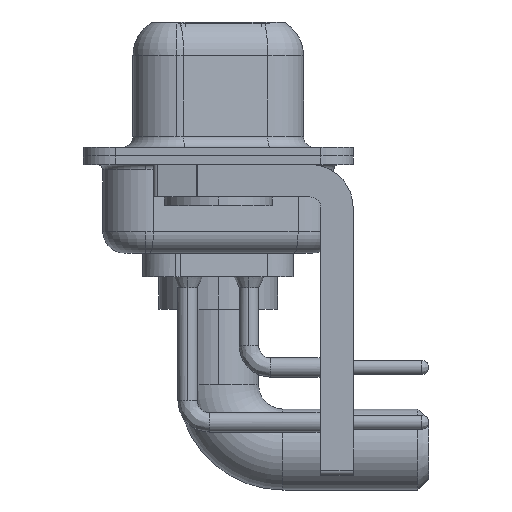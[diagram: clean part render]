
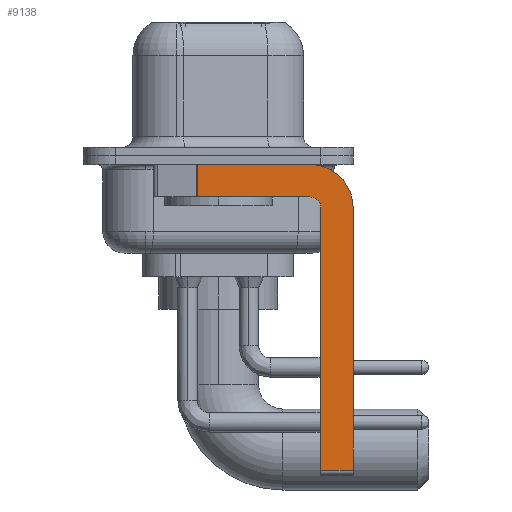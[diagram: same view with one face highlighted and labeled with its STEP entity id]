
A CAD part, left-side view. The second image highlights one B-rep face of the part: STEP entity #9138.
In plain terms, the highlighted planar face has unit normal (-1, 0, 0).
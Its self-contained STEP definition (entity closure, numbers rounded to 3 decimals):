
#435 = CARTESIAN_POINT ( 'NONE',  ( -2.9, -6.25, -2.4 ) ) ;
#586 = AXIS2_PLACEMENT_3D ( 'NONE', #21592, #14474, #12707 ) ;
#688 = VECTOR ( 'NONE', #22884, 1000. ) ;
#944 = CARTESIAN_POINT ( 'NONE',  ( -2.9, 0.978, -1.9 ) ) ;
#1614 = VERTEX_POINT ( 'NONE', #435 ) ;
#1629 = EDGE_CURVE ( 'NONE', #1614, #20230, #9547, .T. ) ;
#2034 = CARTESIAN_POINT ( 'NONE',  ( -2.9, -4.25, -2.4 ) ) ;
#2364 = LINE ( 'NONE', #22265, #22281 ) ;
#2921 = CARTESIAN_POINT ( 'NONE',  ( -2.9, 0.978, -1.9 ) ) ;
#3086 = EDGE_CURVE ( 'NONE', #14313, #6883, #2364, .T. ) ;
#3100 = LINE ( 'NONE', #15648, #688 ) ;
#3863 = CARTESIAN_POINT ( 'NONE',  ( -2.9, -6.25, -2.4 ) ) ;
#4232 = ORIENTED_EDGE ( 'NONE', *, *, #3086, .F. ) ;
#4693 = DIRECTION ( 'NONE',  ( 0., -1., 0. ) ) ;
#4716 = ORIENTED_EDGE ( 'NONE', *, *, #12273, .F. ) ;
#4939 = CARTESIAN_POINT ( 'NONE',  ( -2.9, -4.25, -14.55 ) ) ;
#5197 = CIRCLE ( 'NONE', #21853, 2. ) ;
#5998 = DIRECTION ( 'NONE',  ( 0., 0., -1. ) ) ;
#6318 = EDGE_CURVE ( 'NONE', #11591, #14414, #12734, .T. ) ;
#6357 = CARTESIAN_POINT ( 'NONE',  ( -2.9, 0.978, -0.4 ) ) ;
#6883 = VERTEX_POINT ( 'NONE', #15185 ) ;
#7040 = CARTESIAN_POINT ( 'NONE',  ( -2.9, -4.25, -1.9 ) ) ;
#7110 = AXIS2_PLACEMENT_3D ( 'NONE', #2034, #9254, #7489 ) ;
#7371 = VECTOR ( 'NONE', #9440, 1000. ) ;
#7489 = DIRECTION ( 'NONE',  ( 0., 0., 1. ) ) ;
#7573 = CARTESIAN_POINT ( 'NONE',  ( -2.9, -4.75, -14.55 ) ) ;
#7605 = EDGE_CURVE ( 'NONE', #14313, #14414, #9942, .T. ) ;
#8530 = EDGE_CURVE ( 'NONE', #14307, #11591, #12402, .T. ) ;
#9138 = ADVANCED_FACE ( 'NONE', ( #16151 ), #14369, .F. ) ;
#9254 = DIRECTION ( 'NONE',  ( -1., 0., 0. ) ) ;
#9440 = DIRECTION ( 'NONE',  ( 0., 1., 0. ) ) ;
#9455 = ORIENTED_EDGE ( 'NONE', *, *, #10860, .F. ) ;
#9519 = VERTEX_POINT ( 'NONE', #7573 ) ;
#9547 = LINE ( 'NONE', #3863, #20745 ) ;
#9942 = LINE ( 'NONE', #944, #23328 ) ;
#10139 = EDGE_LOOP ( 'NONE', ( #4232, #22331, #16181, #12250, #9455, #12222, #22493, #4716 ) ) ;
#10860 = EDGE_CURVE ( 'NONE', #9519, #14307, #3100, .T. ) ;
#11591 = VERTEX_POINT ( 'NONE', #7040 ) ;
#11693 = CARTESIAN_POINT ( 'NONE',  ( -2.9, -4.75, -2.4 ) ) ;
#12222 = ORIENTED_EDGE ( 'NONE', *, *, #22833, .T. ) ;
#12250 = ORIENTED_EDGE ( 'NONE', *, *, #8530, .F. ) ;
#12273 = EDGE_CURVE ( 'NONE', #6883, #1614, #5197, .T. ) ;
#12402 = CIRCLE ( 'NONE', #7110, 0.5 ) ;
#12707 = DIRECTION ( 'NONE',  ( 0., 0., -1. ) ) ;
#12734 = LINE ( 'NONE', #21982, #7371 ) ;
#13259 = DIRECTION ( 'NONE',  ( 0., -1., 0. ) ) ;
#13646 = DIRECTION ( 'NONE',  ( 1., 0., 0. ) ) ;
#14307 = VERTEX_POINT ( 'NONE', #11693 ) ;
#14313 = VERTEX_POINT ( 'NONE', #6357 ) ;
#14369 = PLANE ( 'NONE',  #586 ) ;
#14414 = VERTEX_POINT ( 'NONE', #2921 ) ;
#14474 = DIRECTION ( 'NONE',  ( 1., 0., 0. ) ) ;
#14510 = CARTESIAN_POINT ( 'NONE',  ( -2.9, -6.25, -14.55 ) ) ;
#15185 = CARTESIAN_POINT ( 'NONE',  ( -2.9, -4.25, -0.4 ) ) ;
#15614 = DIRECTION ( 'NONE',  ( 0., 0., -1. ) ) ;
#15648 = CARTESIAN_POINT ( 'NONE',  ( -2.9, -4.75, -14.8 ) ) ;
#16151 = FACE_OUTER_BOUND ( 'NONE', #10139, .T. ) ;
#16181 = ORIENTED_EDGE ( 'NONE', *, *, #6318, .F. ) ;
#17606 = LINE ( 'NONE', #4939, #18747 ) ;
#18747 = VECTOR ( 'NONE', #4693, 1000. ) ;
#20230 = VERTEX_POINT ( 'NONE', #14510 ) ;
#20745 = VECTOR ( 'NONE', #5998, 1000. ) ;
#20852 = DIRECTION ( 'NONE',  ( 0., 0., -1. ) ) ;
#21592 = CARTESIAN_POINT ( 'NONE',  ( -2.9, -4.25, -2.4 ) ) ;
#21853 = AXIS2_PLACEMENT_3D ( 'NONE', #22652, #13646, #20852 ) ;
#21982 = CARTESIAN_POINT ( 'NONE',  ( -2.9, -4.25, -1.9 ) ) ;
#22265 = CARTESIAN_POINT ( 'NONE',  ( -2.9, 3., -0.4 ) ) ;
#22281 = VECTOR ( 'NONE', #13259, 1000. ) ;
#22331 = ORIENTED_EDGE ( 'NONE', *, *, #7605, .T. ) ;
#22493 = ORIENTED_EDGE ( 'NONE', *, *, #1629, .F. ) ;
#22652 = CARTESIAN_POINT ( 'NONE',  ( -2.9, -4.25, -2.4 ) ) ;
#22833 = EDGE_CURVE ( 'NONE', #9519, #20230, #17606, .T. ) ;
#22884 = DIRECTION ( 'NONE',  ( 0., 0., 1. ) ) ;
#23328 = VECTOR ( 'NONE', #15614, 1000. ) ;
